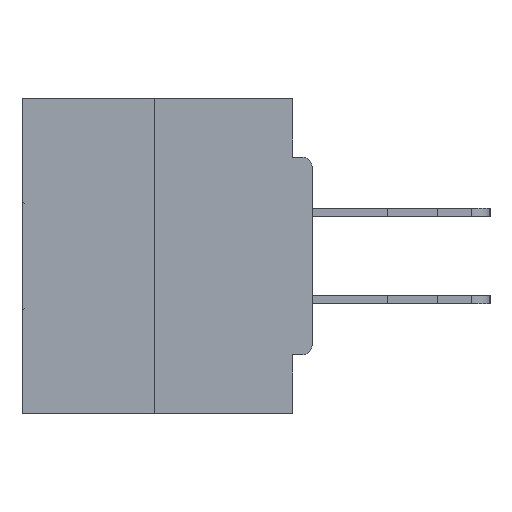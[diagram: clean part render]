
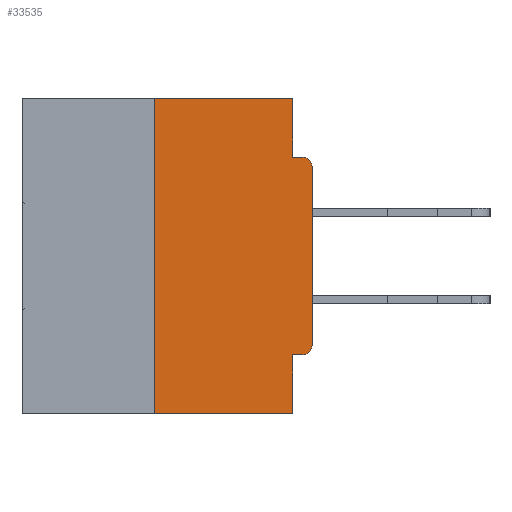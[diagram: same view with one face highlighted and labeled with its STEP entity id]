
A CAD part, left-side view. The second image highlights one B-rep face of the part: STEP entity #33535.
In plain terms, the highlighted planar face has unit normal (-1, 0, 0).
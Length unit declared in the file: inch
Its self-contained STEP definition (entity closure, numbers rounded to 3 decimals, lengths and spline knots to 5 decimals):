
#133 = EDGE_CURVE ( 'NONE', #28344, #35741, #5957, .T. ) ;
#166 = LINE ( 'NONE', #38253, #33280 ) ;
#1025 = DIRECTION ( 'NONE',  ( 0., 1., 0. ) ) ;
#1539 = DIRECTION ( 'NONE',  ( 0., -1., 0. ) ) ;
#1690 = EDGE_CURVE ( 'NONE', #24725, #11818, #11077, .T. ) ;
#3513 = VECTOR ( 'NONE', #32608, 39.37008 ) ;
#3578 = CARTESIAN_POINT ( 'NONE',  ( 0., 0.46, 0. ) ) ;
#3996 = DIRECTION ( 'NONE',  ( 0., 0., -1. ) ) ;
#4313 = EDGE_CURVE ( 'NONE', #32840, #11818, #13030, .T. ) ;
#4530 = DIRECTION ( 'NONE',  ( 0., 0., 1. ) ) ;
#4664 = LINE ( 'NONE', #17343, #33687 ) ;
#4815 = VERTEX_POINT ( 'NONE', #32367 ) ;
#5957 = CIRCLE ( 'NONE', #25204, 0.015 ) ;
#6429 = EDGE_CURVE ( 'NONE', #35741, #14334, #14106, .T. ) ;
#6768 = VECTOR ( 'NONE', #4530, 39.37008 ) ;
#7116 = FACE_OUTER_BOUND ( 'NONE', #33768, .T. ) ;
#7425 = CARTESIAN_POINT ( 'NONE',  ( 0., 0.25, 0. ) ) ;
#7797 = VECTOR ( 'NONE', #29736, 39.37008 ) ;
#9176 = ORIENTED_EDGE ( 'NONE', *, *, #6429, .T. ) ;
#10101 = AXIS2_PLACEMENT_3D ( 'NONE', #3578, #32527, #3996 ) ;
#10242 = VECTOR ( 'NONE', #1025, 39.37008 ) ;
#10788 = CARTESIAN_POINT ( 'NONE',  ( 0., 0.25, -0.5 ) ) ;
#11077 = LINE ( 'NONE', #26502, #30199 ) ;
#11818 = VERTEX_POINT ( 'NONE', #21114 ) ;
#12597 = ORIENTED_EDGE ( 'NONE', *, *, #19018, .T. ) ;
#12835 = DIRECTION ( 'NONE',  ( 0., -1., 0. ) ) ;
#13030 = LINE ( 'NONE', #32204, #29562 ) ;
#13231 = LINE ( 'NONE', #19898, #3513 ) ;
#14106 = LINE ( 'NONE', #16404, #7797 ) ;
#14334 = VERTEX_POINT ( 'NONE', #40089 ) ;
#14490 = VERTEX_POINT ( 'NONE', #24879 ) ;
#15254 = CARTESIAN_POINT ( 'NONE',  ( 0., 0.031, -0.0935 ) ) ;
#15443 = ORIENTED_EDGE ( 'NONE', *, *, #34279, .F. ) ;
#16404 = CARTESIAN_POINT ( 'NONE',  ( 0., 0., 0. ) ) ;
#16888 = PLANE ( 'NONE',  #10101 ) ;
#17059 = DIRECTION ( 'NONE',  ( -1., 0., 0. ) ) ;
#17343 = CARTESIAN_POINT ( 'NONE',  ( 0., 0.46, 0. ) ) ;
#18324 = ORIENTED_EDGE ( 'NONE', *, *, #1690, .F. ) ;
#18968 = CARTESIAN_POINT ( 'NONE',  ( 0., 0.015, -0.4065 ) ) ;
#19018 = EDGE_CURVE ( 'NONE', #14334, #14490, #21231, .T. ) ;
#19175 = ORIENTED_EDGE ( 'NONE', *, *, #4313, .T. ) ;
#19898 = CARTESIAN_POINT ( 'NONE',  ( 0., 0.031, 0. ) ) ;
#19969 = CARTESIAN_POINT ( 'NONE',  ( 0., 0., -0.4065 ) ) ;
#20185 = CARTESIAN_POINT ( 'NONE',  ( 0., 0.015, -0.3915 ) ) ;
#20481 = EDGE_CURVE ( 'NONE', #35462, #14490, #166, .T. ) ;
#20806 = CARTESIAN_POINT ( 'NONE',  ( 0., 0., -0.3915 ) ) ;
#21114 = CARTESIAN_POINT ( 'NONE',  ( 0., 0.031, -0.5 ) ) ;
#21231 = CIRCLE ( 'NONE', #23899, 0.015 ) ;
#23712 = DIRECTION ( 'NONE',  ( -1., 0., 0. ) ) ;
#23807 = DIRECTION ( 'NONE',  ( 0., 0., -1. ) ) ;
#23899 = AXIS2_PLACEMENT_3D ( 'NONE', #26832, #23712, #36423 ) ;
#23955 = ORIENTED_EDGE ( 'NONE', *, *, #37341, .F. ) ;
#24725 = VERTEX_POINT ( 'NONE', #28043 ) ;
#24879 = CARTESIAN_POINT ( 'NONE',  ( 0., 0.015, -0.0935 ) ) ;
#25204 = AXIS2_PLACEMENT_3D ( 'NONE', #20185, #17059, #38729 ) ;
#26502 = CARTESIAN_POINT ( 'NONE',  ( 0., 0.031, -0.5 ) ) ;
#26832 = CARTESIAN_POINT ( 'NONE',  ( 0., 0.015, -0.1085 ) ) ;
#27508 = ORIENTED_EDGE ( 'NONE', *, *, #133, .T. ) ;
#28043 = CARTESIAN_POINT ( 'NONE',  ( 0., 0.031, -0.4065 ) ) ;
#28344 = VERTEX_POINT ( 'NONE', #18968 ) ;
#29329 = EDGE_CURVE ( 'NONE', #32840, #4815, #33059, .T. ) ;
#29346 = LINE ( 'NONE', #19969, #10242 ) ;
#29562 = VECTOR ( 'NONE', #37105, 39.37008 ) ;
#29736 = DIRECTION ( 'NONE',  ( 0., 0., 1. ) ) ;
#30199 = VECTOR ( 'NONE', #23807, 39.37008 ) ;
#31245 = VERTEX_POINT ( 'NONE', #31428 ) ;
#31428 = CARTESIAN_POINT ( 'NONE',  ( 0., 0.031, 0. ) ) ;
#32204 = CARTESIAN_POINT ( 'NONE',  ( 0., 0.46, -0.5 ) ) ;
#32367 = CARTESIAN_POINT ( 'NONE',  ( 0., 0.25, 0. ) ) ;
#32527 = DIRECTION ( 'NONE',  ( 1., 0., 0. ) ) ;
#32608 = DIRECTION ( 'NONE',  ( 0., 0., -1. ) ) ;
#32840 = VERTEX_POINT ( 'NONE', #10788 ) ;
#33059 = LINE ( 'NONE', #7425, #6768 ) ;
#33280 = VECTOR ( 'NONE', #12835, 39.37008 ) ;
#33535 = ADVANCED_FACE ( 'NONE', ( #7116 ), #16888, .F. ) ;
#33687 = VECTOR ( 'NONE', #1539, 39.37008 ) ;
#33768 = EDGE_LOOP ( 'NONE', ( #37743, #34400, #19175, #18324, #23955, #27508, #9176, #12597, #39573, #15443 ) ) ;
#34279 = EDGE_CURVE ( 'NONE', #31245, #35462, #13231, .T. ) ;
#34400 = ORIENTED_EDGE ( 'NONE', *, *, #29329, .F. ) ;
#35462 = VERTEX_POINT ( 'NONE', #15254 ) ;
#35741 = VERTEX_POINT ( 'NONE', #20806 ) ;
#36423 = DIRECTION ( 'NONE',  ( 0., 0., -1. ) ) ;
#37105 = DIRECTION ( 'NONE',  ( 0., -1., 0. ) ) ;
#37341 = EDGE_CURVE ( 'NONE', #28344, #24725, #29346, .T. ) ;
#37743 = ORIENTED_EDGE ( 'NONE', *, *, #38864, .F. ) ;
#38253 = CARTESIAN_POINT ( 'NONE',  ( 0., 0., -0.0935 ) ) ;
#38729 = DIRECTION ( 'NONE',  ( 0., 0., -1. ) ) ;
#38864 = EDGE_CURVE ( 'NONE', #4815, #31245, #4664, .T. ) ;
#39573 = ORIENTED_EDGE ( 'NONE', *, *, #20481, .F. ) ;
#40089 = CARTESIAN_POINT ( 'NONE',  ( 0., 0., -0.1085 ) ) ;
